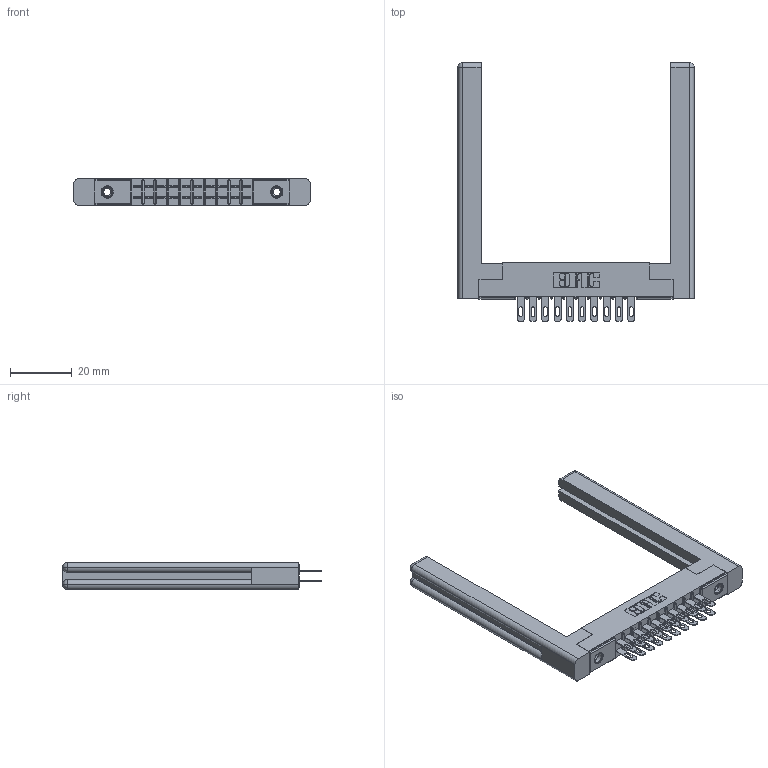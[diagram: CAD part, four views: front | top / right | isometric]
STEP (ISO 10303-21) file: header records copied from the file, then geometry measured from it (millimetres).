
FILE_DESCRIPTION (( 'STEP AP203' ), '1' );
FILE_NAME ('355-020-500-558.STEP', '2019-09-11T03:11:26', ( '' ), ( '' ), 'SwSTEP 2.0', 'SolidWorks 2016', '' );
FILE_SCHEMA (( 'CONFIG_CONTROL_DESIGN' ));
Length unit declared in the file: inch
Products named in the file (5): 307-220-058; 345-250-001_345-250-001-102; 305-290-001_500; 355-020-500-558; 305 Part_.156 Dia
Assembly tree (25 placements, depth 2):
  355-020-500-558
    305 Part_.156 Dia
    305-290-001_500  x20
    345-250-001_345-250-001-102  x2
    307-220-058  x2
Bounding box: 76.25 x 83.49 x 8.71 mm (x, y, z)
Volume: 12439.7 mm3; surface area: 13934.5 mm2
Topology: 25 solids, 25 shells, 1258 faces, 3540 edges, 2292 vertices
Faces by surface type: plane 712, cylinder 482, sphere 40, cone 12, torus 12
Entity records: 17378 total; most frequent: CARTESIAN_POINT 2891, ORIENTED_EDGE 2806, DIRECTION 2787, EDGE_CURVE 1403, VECTOR 1087, LINE 1087, VERTEX_POINT 900, AXIS2_PLACEMENT_3D 850
